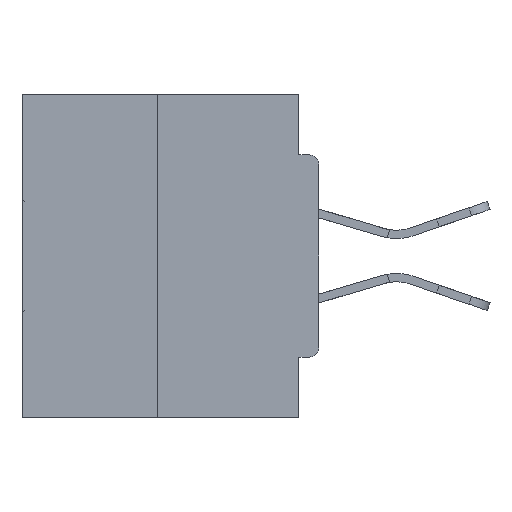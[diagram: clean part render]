
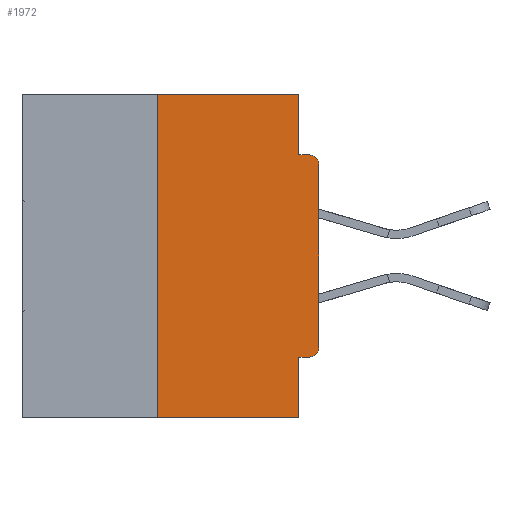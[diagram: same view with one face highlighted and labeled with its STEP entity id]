
A CAD part, left-side view. The second image highlights one B-rep face of the part: STEP entity #1972.
In plain terms, the highlighted planar face has unit normal (-1, 0, 0).
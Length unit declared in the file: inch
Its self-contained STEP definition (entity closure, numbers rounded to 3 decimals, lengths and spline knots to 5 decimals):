
#241 = CARTESIAN_POINT ( 'NONE',  ( 0., 0.25, 0. ) ) ;
#951 = CIRCLE ( 'NONE', #8169, 0.015 ) ;
#1160 = DIRECTION ( 'NONE',  ( 0., 0., -1. ) ) ;
#1972 = ADVANCED_FACE ( 'NONE', ( #34056 ), #34436, .F. ) ;
#2153 = CARTESIAN_POINT ( 'NONE',  ( 0., 0., -0.0935 ) ) ;
#2483 = EDGE_CURVE ( 'NONE', #21027, #20829, #24800, .T. ) ;
#2617 = ORIENTED_EDGE ( 'NONE', *, *, #2483, .F. ) ;
#2987 = CARTESIAN_POINT ( 'NONE',  ( 0., 0.015, -0.4065 ) ) ;
#3705 = VECTOR ( 'NONE', #23200, 39.37008 ) ;
#4505 = ORIENTED_EDGE ( 'NONE', *, *, #6543, .F. ) ;
#4590 = CARTESIAN_POINT ( 'NONE',  ( 0., 0., -0.1085 ) ) ;
#4646 = CARTESIAN_POINT ( 'NONE',  ( 0., 0.031, -0.5 ) ) ;
#4774 = VECTOR ( 'NONE', #15140, 39.37008 ) ;
#6327 = CARTESIAN_POINT ( 'NONE',  ( 0., 0.031, 0. ) ) ;
#6367 = VECTOR ( 'NONE', #14852, 39.37008 ) ;
#6543 = EDGE_CURVE ( 'NONE', #14054, #21027, #26177, .T. ) ;
#7122 = EDGE_CURVE ( 'NONE', #14054, #31423, #951, .T. ) ;
#7727 = ORIENTED_EDGE ( 'NONE', *, *, #19969, .F. ) ;
#8127 = LINE ( 'NONE', #35729, #35852 ) ;
#8169 = AXIS2_PLACEMENT_3D ( 'NONE', #32899, #14283, #1160 ) ;
#8538 = ORIENTED_EDGE ( 'NONE', *, *, #26040, .F. ) ;
#8644 = CARTESIAN_POINT ( 'NONE',  ( 0., 0.031, -0.0935 ) ) ;
#8670 = EDGE_LOOP ( 'NONE', ( #7727, #8877, #39059, #2617, #4505, #9661, #37033, #31355, #35831, #8538 ) ) ;
#8733 = CARTESIAN_POINT ( 'NONE',  ( 0., 0.46, 0. ) ) ;
#8877 = ORIENTED_EDGE ( 'NONE', *, *, #12260, .F. ) ;
#9661 = ORIENTED_EDGE ( 'NONE', *, *, #7122, .T. ) ;
#11295 = CARTESIAN_POINT ( 'NONE',  ( 0., 0.25, -0.5 ) ) ;
#11517 = VERTEX_POINT ( 'NONE', #4590 ) ;
#11791 = DIRECTION ( 'NONE',  ( 0., 0., -1. ) ) ;
#12260 = EDGE_CURVE ( 'NONE', #31593, #33328, #39757, .T. ) ;
#13010 = VERTEX_POINT ( 'NONE', #8644 ) ;
#14054 = VERTEX_POINT ( 'NONE', #2987 ) ;
#14283 = DIRECTION ( 'NONE',  ( -1., 0., 0. ) ) ;
#14852 = DIRECTION ( 'NONE',  ( 0., -1., 0. ) ) ;
#15140 = DIRECTION ( 'NONE',  ( 0., 0., 1. ) ) ;
#15187 = CARTESIAN_POINT ( 'NONE',  ( 0., 0.031, 0. ) ) ;
#16482 = DIRECTION ( 'NONE',  ( 0., -1., 0. ) ) ;
#16890 = VERTEX_POINT ( 'NONE', #6327 ) ;
#18241 = DIRECTION ( 'NONE',  ( 1., 0., 0. ) ) ;
#18442 = LINE ( 'NONE', #38715, #28137 ) ;
#19969 = EDGE_CURVE ( 'NONE', #33328, #16890, #8127, .T. ) ;
#20313 = DIRECTION ( 'NONE',  ( -1., 0., 0. ) ) ;
#20829 = VERTEX_POINT ( 'NONE', #4646 ) ;
#21027 = VERTEX_POINT ( 'NONE', #23665 ) ;
#22159 = EDGE_CURVE ( 'NONE', #31593, #20829, #18442, .T. ) ;
#22415 = EDGE_CURVE ( 'NONE', #13010, #34371, #27905, .T. ) ;
#22493 = DIRECTION ( 'NONE',  ( 0., -1., 0. ) ) ;
#23200 = DIRECTION ( 'NONE',  ( 0., 0., -1. ) ) ;
#23665 = CARTESIAN_POINT ( 'NONE',  ( 0., 0.031, -0.4065 ) ) ;
#24173 = DIRECTION ( 'NONE',  ( 0., 0., -1. ) ) ;
#24269 = CARTESIAN_POINT ( 'NONE',  ( 0., 0.015, -0.0935 ) ) ;
#24800 = LINE ( 'NONE', #42633, #3705 ) ;
#26040 = EDGE_CURVE ( 'NONE', #16890, #13010, #40506, .T. ) ;
#26177 = LINE ( 'NONE', #38825, #37000 ) ;
#26993 = LINE ( 'NONE', #33159, #31603 ) ;
#27013 = CARTESIAN_POINT ( 'NONE',  ( 0., 0., -0.3915 ) ) ;
#27489 = EDGE_CURVE ( 'NONE', #31423, #11517, #26993, .T. ) ;
#27905 = LINE ( 'NONE', #2153, #6367 ) ;
#28137 = VECTOR ( 'NONE', #22493, 39.37008 ) ;
#29863 = EDGE_CURVE ( 'NONE', #11517, #34371, #30695, .T. ) ;
#30695 = CIRCLE ( 'NONE', #32934, 0.015 ) ;
#31355 = ORIENTED_EDGE ( 'NONE', *, *, #29863, .T. ) ;
#31423 = VERTEX_POINT ( 'NONE', #27013 ) ;
#31593 = VERTEX_POINT ( 'NONE', #11295 ) ;
#31603 = VECTOR ( 'NONE', #36624, 39.37008 ) ;
#32330 = DIRECTION ( 'NONE',  ( 0., 1., 0. ) ) ;
#32899 = CARTESIAN_POINT ( 'NONE',  ( 0., 0.015, -0.3915 ) ) ;
#32934 = AXIS2_PLACEMENT_3D ( 'NONE', #36661, #20313, #24173 ) ;
#33159 = CARTESIAN_POINT ( 'NONE',  ( 0., 0., 0. ) ) ;
#33328 = VERTEX_POINT ( 'NONE', #241 ) ;
#34056 = FACE_OUTER_BOUND ( 'NONE', #8670, .T. ) ;
#34371 = VERTEX_POINT ( 'NONE', #24269 ) ;
#34436 = PLANE ( 'NONE',  #39033 ) ;
#34770 = CARTESIAN_POINT ( 'NONE',  ( 0., 0.25, 0. ) ) ;
#35729 = CARTESIAN_POINT ( 'NONE',  ( 0., 0.46, 0. ) ) ;
#35831 = ORIENTED_EDGE ( 'NONE', *, *, #22415, .F. ) ;
#35852 = VECTOR ( 'NONE', #16482, 39.37008 ) ;
#36624 = DIRECTION ( 'NONE',  ( 0., 0., 1. ) ) ;
#36661 = CARTESIAN_POINT ( 'NONE',  ( 0., 0.015, -0.1085 ) ) ;
#37000 = VECTOR ( 'NONE', #32330, 39.37008 ) ;
#37033 = ORIENTED_EDGE ( 'NONE', *, *, #27489, .T. ) ;
#38571 = DIRECTION ( 'NONE',  ( 0., 0., -1. ) ) ;
#38715 = CARTESIAN_POINT ( 'NONE',  ( 0., 0.46, -0.5 ) ) ;
#38825 = CARTESIAN_POINT ( 'NONE',  ( 0., 0., -0.4065 ) ) ;
#39033 = AXIS2_PLACEMENT_3D ( 'NONE', #8733, #18241, #11791 ) ;
#39059 = ORIENTED_EDGE ( 'NONE', *, *, #22159, .T. ) ;
#39449 = VECTOR ( 'NONE', #38571, 39.37008 ) ;
#39757 = LINE ( 'NONE', #34770, #4774 ) ;
#40506 = LINE ( 'NONE', #15187, #39449 ) ;
#42633 = CARTESIAN_POINT ( 'NONE',  ( 0., 0.031, -0.5 ) ) ;
